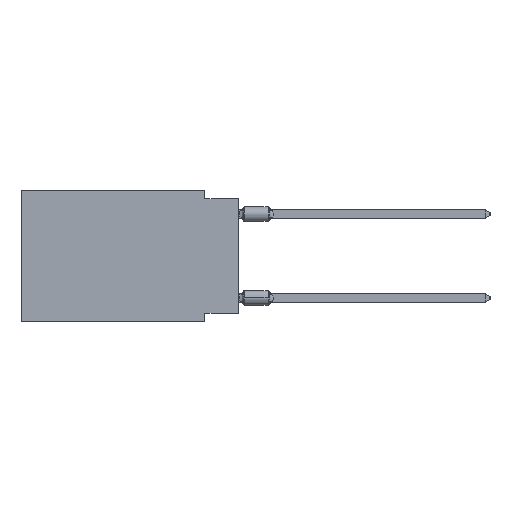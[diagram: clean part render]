
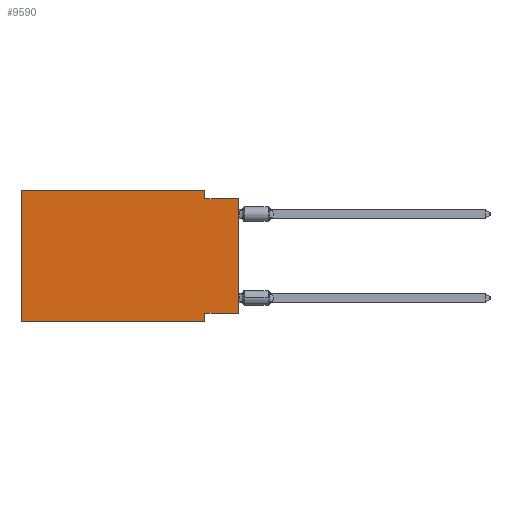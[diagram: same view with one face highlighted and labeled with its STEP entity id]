
A CAD part, left-side view. The second image highlights one B-rep face of the part: STEP entity #9590.
In plain terms, the highlighted planar face has unit normal (-1, 0, 0).
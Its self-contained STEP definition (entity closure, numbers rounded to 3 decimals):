
#88 = VECTOR ( 'NONE', #25032, 1000. ) ;
#610 = LINE ( 'NONE', #15597, #15841 ) ;
#619 = CARTESIAN_POINT ( 'NONE',  ( 0., 2.54, -9.906 ) ) ;
#673 = ORIENTED_EDGE ( 'NONE', *, *, #48253, .F. ) ;
#1352 = ORIENTED_EDGE ( 'NONE', *, *, #42179, .T. ) ;
#1853 = ORIENTED_EDGE ( 'NONE', *, *, #37928, .F. ) ;
#2439 = VERTEX_POINT ( 'NONE', #21578 ) ;
#2538 = CARTESIAN_POINT ( 'NONE',  ( 0., 0., -9.271 ) ) ;
#4986 = VECTOR ( 'NONE', #5445, 1000. ) ;
#5014 = EDGE_CURVE ( 'NONE', #7967, #9755, #29564, .T. ) ;
#5445 = DIRECTION ( 'NONE',  ( 0., 0., -1. ) ) ;
#6092 = CARTESIAN_POINT ( 'NONE',  ( 0., 2.54, -9.906 ) ) ;
#6274 = DIRECTION ( 'NONE',  ( 0., -1., 0. ) ) ;
#6908 = EDGE_CURVE ( 'NONE', #40295, #2439, #30991, .T. ) ;
#7816 = CARTESIAN_POINT ( 'NONE',  ( 0., 0., -0.635 ) ) ;
#7967 = VERTEX_POINT ( 'NONE', #42364 ) ;
#8637 = CARTESIAN_POINT ( 'NONE',  ( 0., 0., -9.271 ) ) ;
#9590 = ADVANCED_FACE ( 'NONE', ( #25861 ), #45097, .F. ) ;
#9755 = VERTEX_POINT ( 'NONE', #619 ) ;
#10616 = DIRECTION ( 'NONE',  ( 0., 0., -1. ) ) ;
#11997 = DIRECTION ( 'NONE',  ( 0., -1., 0. ) ) ;
#13562 = LINE ( 'NONE', #24317, #24218 ) ;
#13977 = CARTESIAN_POINT ( 'NONE',  ( 0., 16.383, -9.906 ) ) ;
#13987 = AXIS2_PLACEMENT_3D ( 'NONE', #48607, #29608, #10616 ) ;
#15597 = CARTESIAN_POINT ( 'NONE',  ( 0., 16.383, 0. ) ) ;
#15841 = VECTOR ( 'NONE', #21937, 1000. ) ;
#19609 = CARTESIAN_POINT ( 'NONE',  ( 0., 16.383, 0. ) ) ;
#20068 = CARTESIAN_POINT ( 'NONE',  ( 0., 0., -0.635 ) ) ;
#21030 = VERTEX_POINT ( 'NONE', #8637 ) ;
#21372 = VERTEX_POINT ( 'NONE', #20068 ) ;
#21578 = CARTESIAN_POINT ( 'NONE',  ( 0., 2.54, 0. ) ) ;
#21937 = DIRECTION ( 'NONE',  ( 0., 0., 1. ) ) ;
#24218 = VECTOR ( 'NONE', #40542, 1000. ) ;
#24317 = CARTESIAN_POINT ( 'NONE',  ( 0., 0., 0. ) ) ;
#25032 = DIRECTION ( 'NONE',  ( 0., 1., 0. ) ) ;
#25861 = FACE_OUTER_BOUND ( 'NONE', #46081, .T. ) ;
#26071 = DIRECTION ( 'NONE',  ( 0., -1., 0. ) ) ;
#26251 = EDGE_CURVE ( 'NONE', #28256, #40295, #610, .T. ) ;
#28256 = VERTEX_POINT ( 'NONE', #13977 ) ;
#28825 = DIRECTION ( 'NONE',  ( 0., 0., -1. ) ) ;
#29268 = LINE ( 'NONE', #36261, #40932 ) ;
#29564 = LINE ( 'NONE', #6092, #47190 ) ;
#29608 = DIRECTION ( 'NONE',  ( 1., 0., 0. ) ) ;
#30991 = LINE ( 'NONE', #46227, #37179 ) ;
#31999 = CARTESIAN_POINT ( 'NONE',  ( 0., 2.54, -0.635 ) ) ;
#32792 = ORIENTED_EDGE ( 'NONE', *, *, #26251, .F. ) ;
#33286 = ORIENTED_EDGE ( 'NONE', *, *, #6908, .F. ) ;
#33954 = ORIENTED_EDGE ( 'NONE', *, *, #39172, .T. ) ;
#34457 = ORIENTED_EDGE ( 'NONE', *, *, #5014, .F. ) ;
#36261 = CARTESIAN_POINT ( 'NONE',  ( 0., 16.383, -9.906 ) ) ;
#36760 = LINE ( 'NONE', #2538, #88 ) ;
#37179 = VECTOR ( 'NONE', #11997, 1000. ) ;
#37405 = ORIENTED_EDGE ( 'NONE', *, *, #48421, .F. ) ;
#37567 = VECTOR ( 'NONE', #26071, 1000. ) ;
#37928 = EDGE_CURVE ( 'NONE', #2439, #40863, #43169, .T. ) ;
#39172 = EDGE_CURVE ( 'NONE', #21030, #21372, #13562, .T. ) ;
#40295 = VERTEX_POINT ( 'NONE', #19609 ) ;
#40542 = DIRECTION ( 'NONE',  ( 0., 0., 1. ) ) ;
#40863 = VERTEX_POINT ( 'NONE', #31999 ) ;
#40932 = VECTOR ( 'NONE', #6274, 1000. ) ;
#42047 = LINE ( 'NONE', #7816, #37567 ) ;
#42179 = EDGE_CURVE ( 'NONE', #28256, #9755, #29268, .T. ) ;
#42364 = CARTESIAN_POINT ( 'NONE',  ( 0., 2.54, -9.271 ) ) ;
#43169 = LINE ( 'NONE', #43424, #4986 ) ;
#43424 = CARTESIAN_POINT ( 'NONE',  ( 0., 2.54, 0. ) ) ;
#45097 = PLANE ( 'NONE',  #13987 ) ;
#46081 = EDGE_LOOP ( 'NONE', ( #33954, #673, #1853, #33286, #32792, #1352, #34457, #37405 ) ) ;
#46227 = CARTESIAN_POINT ( 'NONE',  ( 0., 16.383, 0. ) ) ;
#47190 = VECTOR ( 'NONE', #28825, 1000. ) ;
#48253 = EDGE_CURVE ( 'NONE', #40863, #21372, #42047, .T. ) ;
#48421 = EDGE_CURVE ( 'NONE', #21030, #7967, #36760, .T. ) ;
#48607 = CARTESIAN_POINT ( 'NONE',  ( 0., 16.383, 0. ) ) ;
